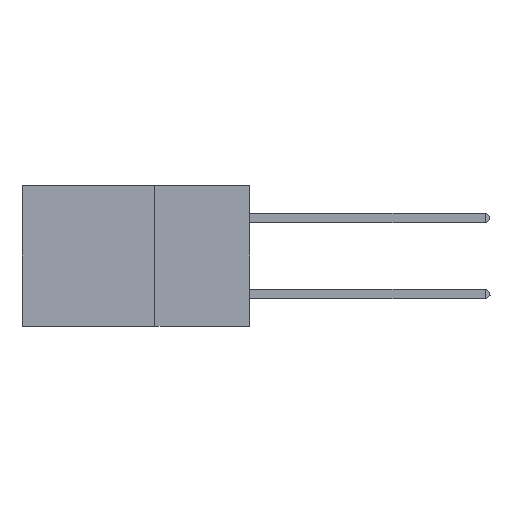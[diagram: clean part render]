
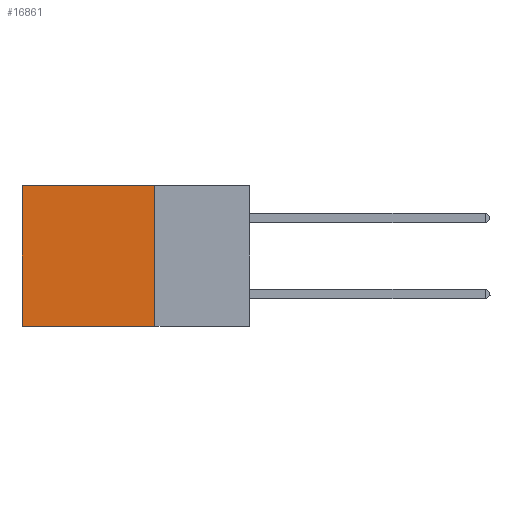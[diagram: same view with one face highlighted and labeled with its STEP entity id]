
A CAD part, left-side view. The second image highlights one B-rep face of the part: STEP entity #16861.
In plain terms, the highlighted planar face has unit normal (-1, 0, 0).
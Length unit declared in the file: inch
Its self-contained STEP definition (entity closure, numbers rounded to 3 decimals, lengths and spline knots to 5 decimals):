
#372 = ORIENTED_EDGE ( 'NONE', *, *, #6166, .F. ) ;
#576 = VERTEX_POINT ( 'NONE', #5585 ) ;
#1137 = DIRECTION ( 'NONE',  ( 0., 1., 0. ) ) ;
#2209 = DIRECTION ( 'NONE',  ( 0., 0., -1. ) ) ;
#2574 = LINE ( 'NONE', #15892, #11552 ) ;
#2731 = AXIS2_PLACEMENT_3D ( 'NONE', #13423, #9222, #14765 ) ;
#2744 = CARTESIAN_POINT ( 'NONE',  ( 0.2875, 0.25, 0. ) ) ;
#3393 = LINE ( 'NONE', #16040, #17232 ) ;
#4041 = LINE ( 'NONE', #6702, #14369 ) ;
#4297 = DIRECTION ( 'NONE',  ( 0., 0., -1. ) ) ;
#5345 = EDGE_LOOP ( 'NONE', ( #10240, #372, #16443, #8713 ) ) ;
#5585 = CARTESIAN_POINT ( 'NONE',  ( 0.2875, 0.25, -0.37 ) ) ;
#6166 = EDGE_CURVE ( 'NONE', #576, #16047, #2574, .T. ) ;
#6195 = FACE_OUTER_BOUND ( 'NONE', #5345, .T. ) ;
#6476 = EDGE_CURVE ( 'NONE', #14670, #16047, #4041, .T. ) ;
#6591 = EDGE_CURVE ( 'NONE', #15133, #14670, #3393, .T. ) ;
#6702 = CARTESIAN_POINT ( 'NONE',  ( 0.2875, 0.6, 0. ) ) ;
#7451 = CARTESIAN_POINT ( 'NONE',  ( 0.2875, 0.25, 0. ) ) ;
#7904 = PLANE ( 'NONE',  #2731 ) ;
#8097 = DIRECTION ( 'NONE',  ( 0., 1., 0. ) ) ;
#8713 = ORIENTED_EDGE ( 'NONE', *, *, #6591, .T. ) ;
#9017 = CARTESIAN_POINT ( 'NONE',  ( 0.2875, 0.6, 0. ) ) ;
#9222 = DIRECTION ( 'NONE',  ( 1., 0., 0. ) ) ;
#9790 = VECTOR ( 'NONE', #2209, 39.37008 ) ;
#10240 = ORIENTED_EDGE ( 'NONE', *, *, #6476, .T. ) ;
#11552 = VECTOR ( 'NONE', #1137, 39.37008 ) ;
#11801 = CARTESIAN_POINT ( 'NONE',  ( 0.2875, 0.6, -0.37 ) ) ;
#13423 = CARTESIAN_POINT ( 'NONE',  ( 0.2875, 0.25, 0. ) ) ;
#13843 = LINE ( 'NONE', #7451, #9790 ) ;
#14369 = VECTOR ( 'NONE', #4297, 39.37008 ) ;
#14670 = VERTEX_POINT ( 'NONE', #9017 ) ;
#14765 = DIRECTION ( 'NONE',  ( 0., 0., -1. ) ) ;
#15133 = VERTEX_POINT ( 'NONE', #2744 ) ;
#15332 = EDGE_CURVE ( 'NONE', #15133, #576, #13843, .T. ) ;
#15892 = CARTESIAN_POINT ( 'NONE',  ( 0.2875, 0.25, -0.37 ) ) ;
#16040 = CARTESIAN_POINT ( 'NONE',  ( 0.2875, 0.25, 0. ) ) ;
#16047 = VERTEX_POINT ( 'NONE', #11801 ) ;
#16443 = ORIENTED_EDGE ( 'NONE', *, *, #15332, .F. ) ;
#16861 = ADVANCED_FACE ( 'NONE', ( #6195 ), #7904, .F. ) ;
#17232 = VECTOR ( 'NONE', #8097, 39.37008 ) ;
